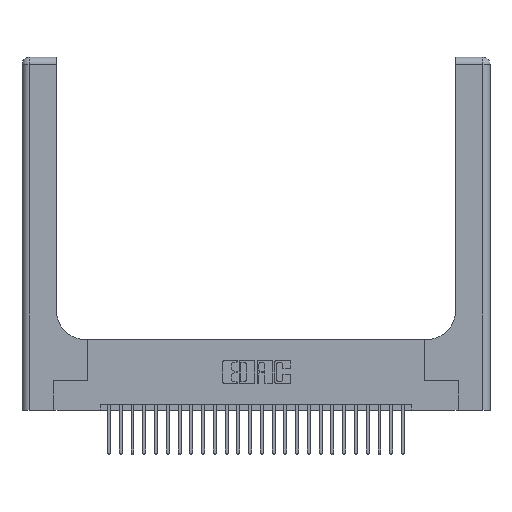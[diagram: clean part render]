
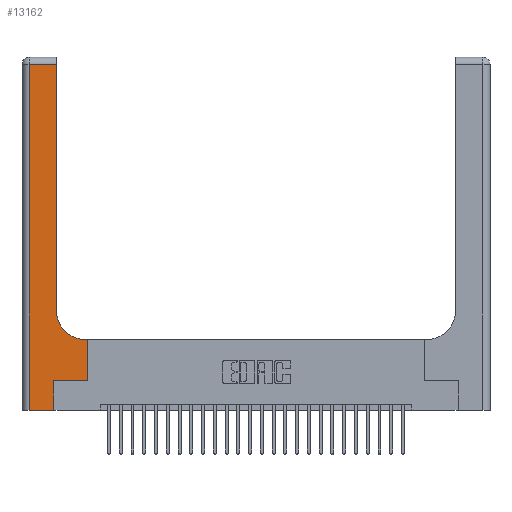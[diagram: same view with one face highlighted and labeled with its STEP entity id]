
A CAD part, top view. The second image highlights one B-rep face of the part: STEP entity #13162.
In plain terms, the highlighted planar face has unit normal (0, 0, 1).
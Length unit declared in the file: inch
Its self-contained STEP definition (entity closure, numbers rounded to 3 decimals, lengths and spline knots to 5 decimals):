
#568 = ORIENTED_EDGE ( 'NONE', *, *, #6811, .T. ) ;
#1510 = VERTEX_POINT ( 'NONE', #25816 ) ;
#1615 = ORIENTED_EDGE ( 'NONE', *, *, #8708, .T. ) ;
#1766 = ORIENTED_EDGE ( 'NONE', *, *, #22657, .T. ) ;
#1826 = DIRECTION ( 'NONE',  ( 1., 0., 0. ) ) ;
#1985 = LINE ( 'NONE', #26111, #17699 ) ;
#3151 = PLANE ( 'NONE',  #16956 ) ;
#3450 = VERTEX_POINT ( 'NONE', #19988 ) ;
#3702 = CARTESIAN_POINT ( 'NONE',  ( 0., 0., 0.37 ) ) ;
#3788 = VECTOR ( 'NONE', #15004, 39.37008 ) ;
#4873 = EDGE_CURVE ( 'NONE', #26875, #18610, #17617, .T. ) ;
#4902 = CARTESIAN_POINT ( 'NONE',  ( 0.5585, 0.25, 0.37 ) ) ;
#5171 = EDGE_CURVE ( 'NONE', #9071, #11097, #16944, .T. ) ;
#6078 = ORIENTED_EDGE ( 'NONE', *, *, #16648, .T. ) ;
#6692 = CARTESIAN_POINT ( 'NONE',  ( 0.2915, 2.94, 0.37 ) ) ;
#6811 = EDGE_CURVE ( 'NONE', #19849, #8887, #7874, .T. ) ;
#6835 = ORIENTED_EDGE ( 'NONE', *, *, #23832, .T. ) ;
#7874 = LINE ( 'NONE', #26155, #15537 ) ;
#8223 = CARTESIAN_POINT ( 'NONE',  ( 0.2915, 3., 0.37 ) ) ;
#8293 = DIRECTION ( 'NONE',  ( 0., -1., 0. ) ) ;
#8553 = LINE ( 'NONE', #10741, #3788 ) ;
#8708 = EDGE_CURVE ( 'NONE', #8887, #9071, #8553, .T. ) ;
#8713 = AXIS2_PLACEMENT_3D ( 'NONE', #19095, #12784, #27473 ) ;
#8887 = VERTEX_POINT ( 'NONE', #17577 ) ;
#8983 = DIRECTION ( 'NONE',  ( 0., 1., 0. ) ) ;
#9071 = VERTEX_POINT ( 'NONE', #26881 ) ;
#10741 = CARTESIAN_POINT ( 'NONE',  ( 0.269, 0.25, 0.37 ) ) ;
#10822 = DIRECTION ( 'NONE',  ( 0., 1., 0. ) ) ;
#10977 = VECTOR ( 'NONE', #8983, 39.37008 ) ;
#11097 = VERTEX_POINT ( 'NONE', #17733 ) ;
#11437 = EDGE_LOOP ( 'NONE', ( #23754, #6835, #1766, #14272, #568, #1615, #14353, #6078, #17484 ) ) ;
#12154 = VECTOR ( 'NONE', #19284, 39.37008 ) ;
#12784 = DIRECTION ( 'NONE',  ( 0., 0., -1. ) ) ;
#13162 = ADVANCED_FACE ( 'NONE', ( #27724 ), #3151, .F. ) ;
#13646 = CARTESIAN_POINT ( 'NONE',  ( 0.269, 0., 0.37 ) ) ;
#13985 = CIRCLE ( 'NONE', #8713, 0.25 ) ;
#14250 = CARTESIAN_POINT ( 'NONE',  ( 0.06, 2.94, 0.37 ) ) ;
#14272 = ORIENTED_EDGE ( 'NONE', *, *, #27372, .T. ) ;
#14353 = ORIENTED_EDGE ( 'NONE', *, *, #5171, .T. ) ;
#15004 = DIRECTION ( 'NONE',  ( 1., 0., 0. ) ) ;
#15225 = LINE ( 'NONE', #3702, #23963 ) ;
#15537 = VECTOR ( 'NONE', #10822, 39.37008 ) ;
#16095 = LINE ( 'NONE', #20863, #12154 ) ;
#16648 = EDGE_CURVE ( 'NONE', #11097, #1510, #16095, .T. ) ;
#16944 = LINE ( 'NONE', #4902, #10977 ) ;
#16956 = AXIS2_PLACEMENT_3D ( 'NONE', #25342, #27608, #27338 ) ;
#17484 = ORIENTED_EDGE ( 'NONE', *, *, #18998, .T. ) ;
#17577 = CARTESIAN_POINT ( 'NONE',  ( 0.269, 0.25, 0.37 ) ) ;
#17617 = LINE ( 'NONE', #8223, #17973 ) ;
#17699 = VECTOR ( 'NONE', #24217, 39.37008 ) ;
#17733 = CARTESIAN_POINT ( 'NONE',  ( 0.5585, 0.6, 0.37 ) ) ;
#17973 = VECTOR ( 'NONE', #21082, 39.37008 ) ;
#18162 = VECTOR ( 'NONE', #8293, 39.37008 ) ;
#18610 = VERTEX_POINT ( 'NONE', #6692 ) ;
#18648 = CARTESIAN_POINT ( 'NONE',  ( 0.06, 3., 0.37 ) ) ;
#18998 = EDGE_CURVE ( 'NONE', #1510, #26875, #13985, .T. ) ;
#19095 = CARTESIAN_POINT ( 'NONE',  ( 0.5415, 0.85, 0.37 ) ) ;
#19284 = DIRECTION ( 'NONE',  ( -1., 0., 0. ) ) ;
#19720 = CARTESIAN_POINT ( 'NONE',  ( 0.2915, 0.85, 0.37 ) ) ;
#19849 = VERTEX_POINT ( 'NONE', #13646 ) ;
#19988 = CARTESIAN_POINT ( 'NONE',  ( 0.06, 0., 0.37 ) ) ;
#20863 = CARTESIAN_POINT ( 'NONE',  ( 0.2915, 0.6, 0.37 ) ) ;
#21082 = DIRECTION ( 'NONE',  ( 0., 1., 0. ) ) ;
#22657 = EDGE_CURVE ( 'NONE', #24931, #3450, #25909, .T. ) ;
#23754 = ORIENTED_EDGE ( 'NONE', *, *, #4873, .T. ) ;
#23832 = EDGE_CURVE ( 'NONE', #18610, #24931, #1985, .T. ) ;
#23963 = VECTOR ( 'NONE', #1826, 39.37008 ) ;
#24217 = DIRECTION ( 'NONE',  ( -1., 0., 0. ) ) ;
#24931 = VERTEX_POINT ( 'NONE', #14250 ) ;
#25342 = CARTESIAN_POINT ( 'NONE',  ( 0., 3., 0.37 ) ) ;
#25816 = CARTESIAN_POINT ( 'NONE',  ( 0.5415, 0.6, 0.37 ) ) ;
#25909 = LINE ( 'NONE', #18648, #18162 ) ;
#26111 = CARTESIAN_POINT ( 'NONE',  ( 0., 2.94, 0.37 ) ) ;
#26155 = CARTESIAN_POINT ( 'NONE',  ( 0.269, 0., 0.37 ) ) ;
#26875 = VERTEX_POINT ( 'NONE', #19720 ) ;
#26881 = CARTESIAN_POINT ( 'NONE',  ( 0.5585, 0.25, 0.37 ) ) ;
#27338 = DIRECTION ( 'NONE',  ( -1., 0., 0. ) ) ;
#27372 = EDGE_CURVE ( 'NONE', #3450, #19849, #15225, .T. ) ;
#27473 = DIRECTION ( 'NONE',  ( 1., 0., 0. ) ) ;
#27608 = DIRECTION ( 'NONE',  ( 0., 0., -1. ) ) ;
#27724 = FACE_OUTER_BOUND ( 'NONE', #11437, .T. ) ;
